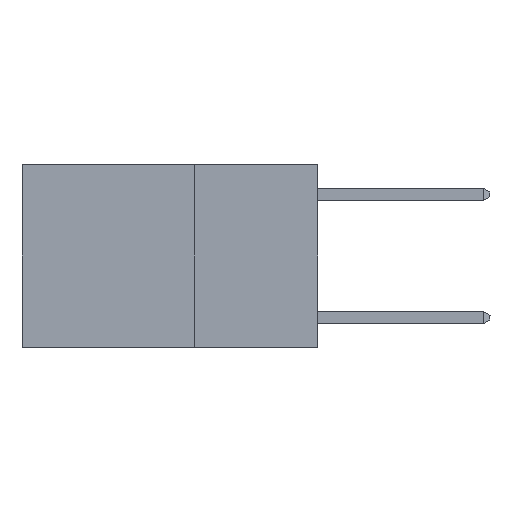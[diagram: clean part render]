
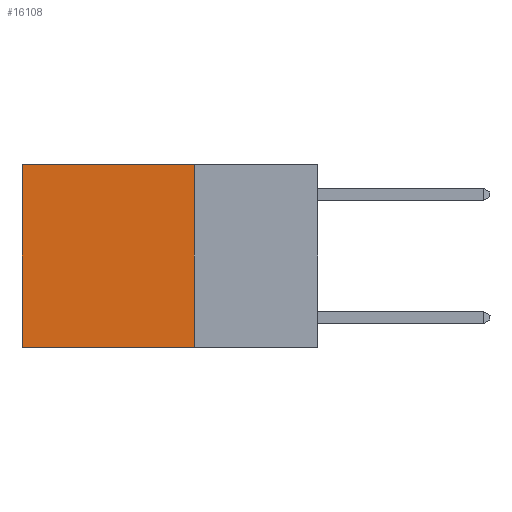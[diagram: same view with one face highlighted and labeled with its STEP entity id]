
A CAD part, left-side view. The second image highlights one B-rep face of the part: STEP entity #16108.
In plain terms, the highlighted planar face has unit normal (-1, 0, 0).
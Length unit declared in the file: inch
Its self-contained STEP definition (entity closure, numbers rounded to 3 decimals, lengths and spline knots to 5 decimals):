
#1056 = FACE_OUTER_BOUND ( 'NONE', #19973, .T. ) ;
#1307 = ORIENTED_EDGE ( 'NONE', *, *, #11996, .F. ) ;
#1465 = LINE ( 'NONE', #9017, #16715 ) ;
#2184 = DIRECTION ( 'NONE',  ( 0., 0., -1. ) ) ;
#2350 = AXIS2_PLACEMENT_3D ( 'NONE', #7839, #23505, #11832 ) ;
#2768 = CARTESIAN_POINT ( 'NONE',  ( 0.2625, 0.25, 0. ) ) ;
#3144 = VERTEX_POINT ( 'NONE', #5218 ) ;
#4033 = CARTESIAN_POINT ( 'NONE',  ( 0.2625, 0.6, -0.37 ) ) ;
#5218 = CARTESIAN_POINT ( 'NONE',  ( 0.2625, 0.25, -0.37 ) ) ;
#6688 = VERTEX_POINT ( 'NONE', #14465 ) ;
#7839 = CARTESIAN_POINT ( 'NONE',  ( 0.2625, 0.25, 0. ) ) ;
#8117 = EDGE_CURVE ( 'NONE', #12968, #3144, #13496, .T. ) ;
#9017 = CARTESIAN_POINT ( 'NONE',  ( 0.2625, 0.25, 0. ) ) ;
#9923 = VERTEX_POINT ( 'NONE', #4033 ) ;
#11018 = DIRECTION ( 'NONE',  ( 0., 1., 0. ) ) ;
#11069 = CARTESIAN_POINT ( 'NONE',  ( 0.2625, 0.25, 0. ) ) ;
#11386 = VECTOR ( 'NONE', #14367, 39.37008 ) ;
#11832 = DIRECTION ( 'NONE',  ( 0., 0., -1. ) ) ;
#11996 = EDGE_CURVE ( 'NONE', #3144, #9923, #16632, .T. ) ;
#12110 = DIRECTION ( 'NONE',  ( 0., 1., 0. ) ) ;
#12968 = VERTEX_POINT ( 'NONE', #2768 ) ;
#13358 = ORIENTED_EDGE ( 'NONE', *, *, #14484, .T. ) ;
#13496 = LINE ( 'NONE', #11069, #23208 ) ;
#14367 = DIRECTION ( 'NONE',  ( 0., 0., -1. ) ) ;
#14465 = CARTESIAN_POINT ( 'NONE',  ( 0.2625, 0.6, 0. ) ) ;
#14484 = EDGE_CURVE ( 'NONE', #12968, #6688, #1465, .T. ) ;
#14634 = ORIENTED_EDGE ( 'NONE', *, *, #8117, .F. ) ;
#16108 = ADVANCED_FACE ( 'NONE', ( #1056 ), #19651, .F. ) ;
#16283 = EDGE_CURVE ( 'NONE', #6688, #9923, #21208, .T. ) ;
#16632 = LINE ( 'NONE', #19914, #21228 ) ;
#16715 = VECTOR ( 'NONE', #11018, 39.37008 ) ;
#19651 = PLANE ( 'NONE',  #2350 ) ;
#19914 = CARTESIAN_POINT ( 'NONE',  ( 0.2625, 0.25, -0.37 ) ) ;
#19973 = EDGE_LOOP ( 'NONE', ( #24948, #1307, #14634, #13358 ) ) ;
#21208 = LINE ( 'NONE', #23964, #11386 ) ;
#21228 = VECTOR ( 'NONE', #12110, 39.37008 ) ;
#23208 = VECTOR ( 'NONE', #2184, 39.37008 ) ;
#23505 = DIRECTION ( 'NONE',  ( 1., 0., 0. ) ) ;
#23964 = CARTESIAN_POINT ( 'NONE',  ( 0.2625, 0.6, 0. ) ) ;
#24948 = ORIENTED_EDGE ( 'NONE', *, *, #16283, .T. ) ;
